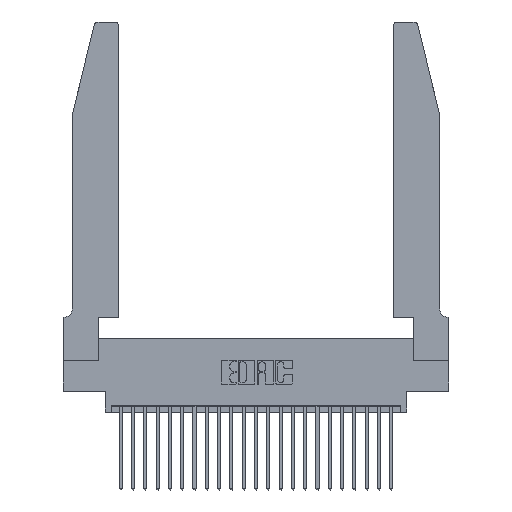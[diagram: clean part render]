
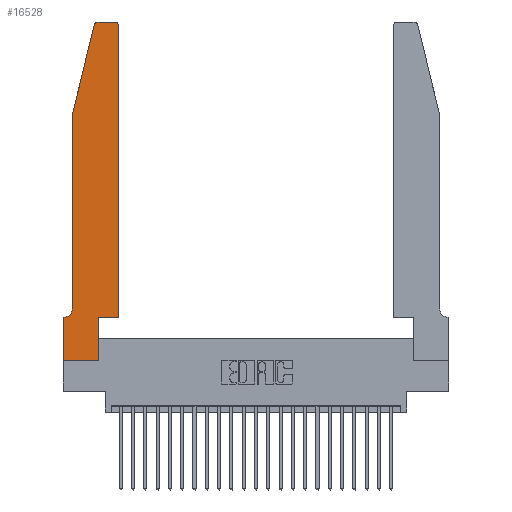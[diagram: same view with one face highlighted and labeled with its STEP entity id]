
A CAD part, top view. The second image highlights one B-rep face of the part: STEP entity #16528.
In plain terms, the highlighted planar face has unit normal (0, 0, 1).
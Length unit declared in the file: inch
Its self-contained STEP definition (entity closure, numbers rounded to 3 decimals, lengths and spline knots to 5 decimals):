
#28 = CARTESIAN_POINT ( 'NONE',  ( 0., 0.35, 0.37 ) ) ;
#81 = LINE ( 'NONE', #22380, #9684 ) ;
#273 = EDGE_LOOP ( 'NONE', ( #7259, #7342, #7465, #7735, #7765, #7955, #8025, #8228, #8284, #8364, #8589, #8996 ) ) ;
#467 = DIRECTION ( 'NONE',  ( 1., 0., 0. ) ) ;
#504 = DIRECTION ( 'NONE',  ( 0., 0., 1. ) ) ;
#941 = EDGE_CURVE ( 'NONE', #5050, #9571, #6752, .T. ) ;
#969 = AXIS2_PLACEMENT_3D ( 'NONE', #2172, #16167, #4241 ) ;
#1256 = DIRECTION ( 'NONE',  ( 0., 1., 0. ) ) ;
#1632 = DIRECTION ( 'NONE',  ( 0., -1., 0. ) ) ;
#1788 = VERTEX_POINT ( 'NONE', #28 ) ;
#1806 = EDGE_CURVE ( 'NONE', #15247, #5050, #25272, .T. ) ;
#2172 = CARTESIAN_POINT ( 'NONE',  ( 0.0055, 0.42, 0.37 ) ) ;
#2463 = PLANE ( 'NONE',  #4417 ) ;
#3372 = CARTESIAN_POINT ( 'NONE',  ( 0.2605, 2.75, 0.37 ) ) ;
#4073 = EDGE_CURVE ( 'NONE', #18790, #24659, #21346, .T. ) ;
#4241 = DIRECTION ( 'NONE',  ( -1., 0., 0. ) ) ;
#4393 = EDGE_CURVE ( 'NONE', #1788, #6765, #23125, .T. ) ;
#4417 = AXIS2_PLACEMENT_3D ( 'NONE', #14625, #4616, #18476 ) ;
#4431 = LINE ( 'NONE', #3372, #18977 ) ;
#4616 = DIRECTION ( 'NONE',  ( 0., 0., 1. ) ) ;
#4677 = DIRECTION ( 'NONE',  ( 1., 0., 0. ) ) ;
#4742 = DIRECTION ( 'NONE',  ( 0., -1., 0. ) ) ;
#4955 = CARTESIAN_POINT ( 'NONE',  ( 0.0055, 0.35, 0.37 ) ) ;
#5050 = VERTEX_POINT ( 'NONE', #20410 ) ;
#5401 = DIRECTION ( 'NONE',  ( -1., 0., 0. ) ) ;
#5833 = CARTESIAN_POINT ( 'NONE',  ( 0.0755, 2., 0.37 ) ) ;
#6635 = AXIS2_PLACEMENT_3D ( 'NONE', #12689, #504, #14623 ) ;
#6752 = LINE ( 'NONE', #25193, #17261 ) ;
#6765 = VERTEX_POINT ( 'NONE', #19155 ) ;
#7038 = VERTEX_POINT ( 'NONE', #21901 ) ;
#7089 = EDGE_CURVE ( 'NONE', #9571, #18558, #14204, .T. ) ;
#7259 = ORIENTED_EDGE ( 'NONE', *, *, #7317, .T. ) ;
#7317 = EDGE_CURVE ( 'NONE', #18558, #7038, #4431, .T. ) ;
#7342 = ORIENTED_EDGE ( 'NONE', *, *, #20242, .T. ) ;
#7465 = ORIENTED_EDGE ( 'NONE', *, *, #22693, .T. ) ;
#7565 = VECTOR ( 'NONE', #4742, 39.37008 ) ;
#7735 = ORIENTED_EDGE ( 'NONE', *, *, #4073, .T. ) ;
#7765 = ORIENTED_EDGE ( 'NONE', *, *, #15092, .T. ) ;
#7955 = ORIENTED_EDGE ( 'NONE', *, *, #20572, .T. ) ;
#8025 = ORIENTED_EDGE ( 'NONE', *, *, #4393, .T. ) ;
#8228 = ORIENTED_EDGE ( 'NONE', *, *, #11242, .T. ) ;
#8284 = ORIENTED_EDGE ( 'NONE', *, *, #16071, .T. ) ;
#8364 = ORIENTED_EDGE ( 'NONE', *, *, #1806, .T. ) ;
#8546 = CARTESIAN_POINT ( 'NONE',  ( 0.4205, 2.72, 0.37 ) ) ;
#8549 = LINE ( 'NONE', #10523, #18358 ) ;
#8589 = ORIENTED_EDGE ( 'NONE', *, *, #941, .T. ) ;
#8996 = ORIENTED_EDGE ( 'NONE', *, *, #7089, .T. ) ;
#9571 = VERTEX_POINT ( 'NONE', #18612 ) ;
#9622 = VECTOR ( 'NONE', #18700, 39.37008 ) ;
#9684 = VECTOR ( 'NONE', #4677, 39.37008 ) ;
#9809 = CARTESIAN_POINT ( 'NONE',  ( 0.25487, 2.72718, 0.37 ) ) ;
#10448 = VECTOR ( 'NONE', #1632, 39.37008 ) ;
#10523 = CARTESIAN_POINT ( 'NONE',  ( 0.0755, 2., 0.37 ) ) ;
#10583 = DIRECTION ( 'NONE',  ( 1., 0., 0. ) ) ;
#11242 = EDGE_CURVE ( 'NONE', #6765, #24472, #81, .T. ) ;
#12551 = DIRECTION ( 'NONE',  ( -0.239, -0.971, 0. ) ) ;
#12689 = CARTESIAN_POINT ( 'NONE',  ( 0.284, 2.72, 0.37 ) ) ;
#12813 = CARTESIAN_POINT ( 'NONE',  ( 0., 0., 0.37 ) ) ;
#13143 = CARTESIAN_POINT ( 'NONE',  ( 0.2865, 0.35, 0.37 ) ) ;
#13241 = VECTOR ( 'NONE', #18907, 39.37008 ) ;
#13763 = CARTESIAN_POINT ( 'NONE',  ( 0.0755, 2., 0.37 ) ) ;
#13838 = LINE ( 'NONE', #13143, #13241 ) ;
#14204 = CIRCLE ( 'NONE', #21743, 0.03 ) ;
#14623 = DIRECTION ( 'NONE',  ( 1., 0., 0. ) ) ;
#14625 = CARTESIAN_POINT ( 'NONE',  ( 0., 0.35, 0.37 ) ) ;
#14680 = CARTESIAN_POINT ( 'NONE',  ( 0.2865, 0.35, 0.37 ) ) ;
#14857 = LINE ( 'NONE', #16679, #9622 ) ;
#15092 = EDGE_CURVE ( 'NONE', #24659, #20383, #20778, .T. ) ;
#15247 = VERTEX_POINT ( 'NONE', #14680 ) ;
#16071 = EDGE_CURVE ( 'NONE', #24472, #15247, #13838, .T. ) ;
#16167 = DIRECTION ( 'NONE',  ( 0., 0., -1. ) ) ;
#16528 = ADVANCED_FACE ( 'NONE', ( #18298 ), #2463, .T. ) ;
#16670 = CARTESIAN_POINT ( 'NONE',  ( 0.4505, 0.35, 0.37 ) ) ;
#16679 = CARTESIAN_POINT ( 'NONE',  ( 0.0755, 0.35, 0.37 ) ) ;
#17261 = VECTOR ( 'NONE', #1256, 39.37008 ) ;
#17581 = CIRCLE ( 'NONE', #6635, 0.03 ) ;
#18298 = FACE_OUTER_BOUND ( 'NONE', #273, .T. ) ;
#18358 = VECTOR ( 'NONE', #12551, 39.37008 ) ;
#18476 = DIRECTION ( 'NONE',  ( 1., 0., 0. ) ) ;
#18558 = VERTEX_POINT ( 'NONE', #22396 ) ;
#18612 = CARTESIAN_POINT ( 'NONE',  ( 0.4505, 2.72, 0.37 ) ) ;
#18700 = DIRECTION ( 'NONE',  ( -1., 0., 0. ) ) ;
#18790 = VERTEX_POINT ( 'NONE', #5833 ) ;
#18907 = DIRECTION ( 'NONE',  ( 0., 1., 0. ) ) ;
#18977 = VECTOR ( 'NONE', #5401, 39.37008 ) ;
#19155 = CARTESIAN_POINT ( 'NONE',  ( 0., 0., 0.37 ) ) ;
#20228 = VECTOR ( 'NONE', #467, 39.37008 ) ;
#20242 = EDGE_CURVE ( 'NONE', #7038, #22995, #17581, .T. ) ;
#20383 = VERTEX_POINT ( 'NONE', #4955 ) ;
#20410 = CARTESIAN_POINT ( 'NONE',  ( 0.4505, 0.35, 0.37 ) ) ;
#20572 = EDGE_CURVE ( 'NONE', #20383, #1788, #14857, .T. ) ;
#20778 = CIRCLE ( 'NONE', #969, 0.07 ) ;
#21346 = LINE ( 'NONE', #13763, #10448 ) ;
#21687 = CARTESIAN_POINT ( 'NONE',  ( 0.0755, 0.42, 0.37 ) ) ;
#21743 = AXIS2_PLACEMENT_3D ( 'NONE', #8546, #22148, #10583 ) ;
#21901 = CARTESIAN_POINT ( 'NONE',  ( 0.284, 2.75, 0.37 ) ) ;
#22148 = DIRECTION ( 'NONE',  ( 0., 0., 1. ) ) ;
#22380 = CARTESIAN_POINT ( 'NONE',  ( 0., 0., 0.37 ) ) ;
#22396 = CARTESIAN_POINT ( 'NONE',  ( 0.4205, 2.75, 0.37 ) ) ;
#22693 = EDGE_CURVE ( 'NONE', #22995, #18790, #8549, .T. ) ;
#22995 = VERTEX_POINT ( 'NONE', #9809 ) ;
#23048 = CARTESIAN_POINT ( 'NONE',  ( 0.2865, 0., 0.37 ) ) ;
#23125 = LINE ( 'NONE', #12813, #7565 ) ;
#24472 = VERTEX_POINT ( 'NONE', #23048 ) ;
#24659 = VERTEX_POINT ( 'NONE', #21687 ) ;
#25193 = CARTESIAN_POINT ( 'NONE',  ( 0.4505, 0.35, 0.37 ) ) ;
#25272 = LINE ( 'NONE', #16670, #20228 ) ;
